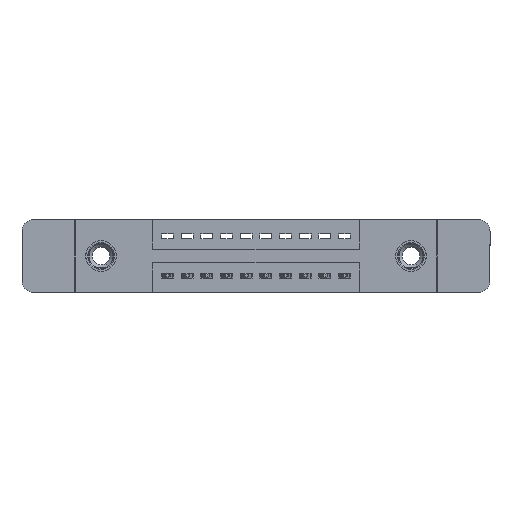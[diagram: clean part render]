
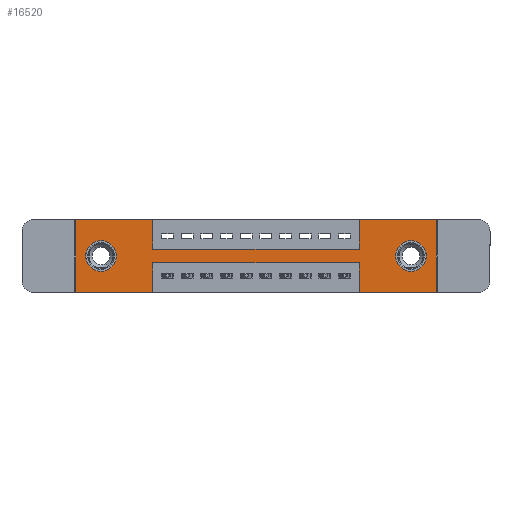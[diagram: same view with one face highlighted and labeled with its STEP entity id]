
A CAD part, front view. The second image highlights one B-rep face of the part: STEP entity #16520.
In plain terms, the highlighted planar face has unit normal (0, -1, 0).
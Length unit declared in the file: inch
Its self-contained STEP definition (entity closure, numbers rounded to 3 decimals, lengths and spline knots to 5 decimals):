
#127 = CARTESIAN_POINT ( 'NONE',  ( 0.3925, 0., 0. ) ) ;
#152 = ORIENTED_EDGE ( 'NONE', *, *, #13595, .F. ) ;
#207 = LINE ( 'NONE', #127, #14600 ) ;
#641 = EDGE_CURVE ( 'NONE', #5445, #3147, #5574, .T. ) ;
#910 = VECTOR ( 'NONE', #4102, 39.37008 ) ;
#1420 = CARTESIAN_POINT ( 'NONE',  ( 0.13, 0., -0.107 ) ) ;
#1727 = ORIENTED_EDGE ( 'NONE', *, *, #8128, .F. ) ;
#1842 = ORIENTED_EDGE ( 'NONE', *, *, #15267, .F. ) ;
#2027 = FACE_BOUND ( 'NONE', #13769, .T. ) ;
#2167 = CARTESIAN_POINT ( 'NONE',  ( 1.4425, 0., -0.37 ) ) ;
#2197 = ORIENTED_EDGE ( 'NONE', *, *, #5052, .F. ) ;
#2280 = VECTOR ( 'NONE', #5036, 39.37008 ) ;
#2352 = CARTESIAN_POINT ( 'NONE',  ( 0., 0., 0. ) ) ;
#2382 = EDGE_CURVE ( 'NONE', #8239, #11735, #10687, .T. ) ;
#2415 = CARTESIAN_POINT ( 'NONE',  ( 0.3925, 0., -0.22 ) ) ;
#2597 = DIRECTION ( 'NONE',  ( -1., 0., 0. ) ) ;
#2602 = VECTOR ( 'NONE', #4194, 39.37008 ) ;
#2706 = EDGE_CURVE ( 'NONE', #8130, #14684, #16845, .T. ) ;
#2824 = CARTESIAN_POINT ( 'NONE',  ( 0., 0., 0. ) ) ;
#2878 = CARTESIAN_POINT ( 'NONE',  ( 1.4425, 0., 0. ) ) ;
#2883 = CARTESIAN_POINT ( 'NONE',  ( 0.3925, 0., -0.37 ) ) ;
#3040 = CARTESIAN_POINT ( 'NONE',  ( 0.3925, 0., 0. ) ) ;
#3147 = VERTEX_POINT ( 'NONE', #8772 ) ;
#3227 = CARTESIAN_POINT ( 'NONE',  ( 1.4425, 0., 0. ) ) ;
#3385 = EDGE_CURVE ( 'NONE', #3861, #8239, #7311, .T. ) ;
#3504 = DIRECTION ( 'NONE',  ( 0., 1., 0. ) ) ;
#3509 = EDGE_CURVE ( 'NONE', #13160, #3861, #6315, .T. ) ;
#3531 = CIRCLE ( 'NONE', #13431, 0.078 ) ;
#3548 = LINE ( 'NONE', #14357, #6642 ) ;
#3686 = VECTOR ( 'NONE', #14288, 39.37008 ) ;
#3698 = ORIENTED_EDGE ( 'NONE', *, *, #14165, .F. ) ;
#3845 = DIRECTION ( 'NONE',  ( 0., 1., 0. ) ) ;
#3861 = VERTEX_POINT ( 'NONE', #3227 ) ;
#3905 = CARTESIAN_POINT ( 'NONE',  ( 1.705, 0., -0.107 ) ) ;
#4102 = DIRECTION ( 'NONE',  ( 1., 0., 0. ) ) ;
#4194 = DIRECTION ( 'NONE',  ( 0., 0., 1. ) ) ;
#4401 = AXIS2_PLACEMENT_3D ( 'NONE', #11737, #3845, #6508 ) ;
#4901 = DIRECTION ( 'NONE',  ( 0., 0., 1. ) ) ;
#4958 = VECTOR ( 'NONE', #14741, 39.37008 ) ;
#5036 = DIRECTION ( 'NONE',  ( 0., 0., 1. ) ) ;
#5052 = EDGE_CURVE ( 'NONE', #11735, #5445, #8006, .T. ) ;
#5140 = CARTESIAN_POINT ( 'NONE',  ( 0.3925, 0., -0.37 ) ) ;
#5337 = CARTESIAN_POINT ( 'NONE',  ( 1.705, 0., -0.263 ) ) ;
#5445 = VERTEX_POINT ( 'NONE', #9207 ) ;
#5574 = LINE ( 'NONE', #2167, #11156 ) ;
#5982 = AXIS2_PLACEMENT_3D ( 'NONE', #14582, #16015, #15901 ) ;
#6210 = CIRCLE ( 'NONE', #4401, 0.078 ) ;
#6250 = VERTEX_POINT ( 'NONE', #3040 ) ;
#6315 = LINE ( 'NONE', #2878, #2602 ) ;
#6354 = ORIENTED_EDGE ( 'NONE', *, *, #2382, .F. ) ;
#6387 = CARTESIAN_POINT ( 'NONE',  ( 0., 0., 0. ) ) ;
#6447 = ORIENTED_EDGE ( 'NONE', *, *, #2706, .F. ) ;
#6468 = DIRECTION ( 'NONE',  ( 0., 1., 0. ) ) ;
#6508 = DIRECTION ( 'NONE',  ( 0., 0., -1. ) ) ;
#6642 = VECTOR ( 'NONE', #2597, 39.37008 ) ;
#7075 = CARTESIAN_POINT ( 'NONE',  ( 0.13, 0., -0.185 ) ) ;
#7215 = LINE ( 'NONE', #2824, #4958 ) ;
#7311 = LINE ( 'NONE', #6387, #10655 ) ;
#7471 = ORIENTED_EDGE ( 'NONE', *, *, #9266, .F. ) ;
#7651 = ORIENTED_EDGE ( 'NONE', *, *, #9530, .T. ) ;
#7866 = EDGE_CURVE ( 'NONE', #9955, #15402, #9528, .T. ) ;
#7925 = DIRECTION ( 'NONE',  ( 0., 0., -1. ) ) ;
#8006 = LINE ( 'NONE', #9879, #11098 ) ;
#8054 = DIRECTION ( 'NONE',  ( 0., 0., -1. ) ) ;
#8111 = AXIS2_PLACEMENT_3D ( 'NONE', #14363, #6468, #9265 ) ;
#8128 = EDGE_CURVE ( 'NONE', #11475, #13160, #12873, .T. ) ;
#8130 = VERTEX_POINT ( 'NONE', #14544 ) ;
#8239 = VERTEX_POINT ( 'NONE', #14656 ) ;
#8362 = EDGE_LOOP ( 'NONE', ( #13503, #11349 ) ) ;
#8706 = VERTEX_POINT ( 'NONE', #12957 ) ;
#8772 = CARTESIAN_POINT ( 'NONE',  ( 1.4425, 0., -0.22 ) ) ;
#9207 = CARTESIAN_POINT ( 'NONE',  ( 1.4425, 0., -0.37 ) ) ;
#9265 = DIRECTION ( 'NONE',  ( 0., 0., 1. ) ) ;
#9266 = EDGE_CURVE ( 'NONE', #14684, #8706, #3548, .T. ) ;
#9275 = VERTEX_POINT ( 'NONE', #5337 ) ;
#9420 = LINE ( 'NONE', #2415, #3686 ) ;
#9528 = CIRCLE ( 'NONE', #8111, 0.078 ) ;
#9530 = EDGE_CURVE ( 'NONE', #12639, #9275, #3531, .T. ) ;
#9879 = CARTESIAN_POINT ( 'NONE',  ( 0., 0., -0.37 ) ) ;
#9925 = VERTEX_POINT ( 'NONE', #14565 ) ;
#9955 = VERTEX_POINT ( 'NONE', #1420 ) ;
#10281 = CARTESIAN_POINT ( 'NONE',  ( 1.4425, 0., -0.15 ) ) ;
#10358 = DIRECTION ( 'NONE',  ( 1., 0., 0. ) ) ;
#10365 = CARTESIAN_POINT ( 'NONE',  ( 1.835, 0., 0. ) ) ;
#10467 = VECTOR ( 'NONE', #8054, 39.37008 ) ;
#10655 = VECTOR ( 'NONE', #10358, 39.37008 ) ;
#10687 = LINE ( 'NONE', #10365, #11513 ) ;
#10866 = CARTESIAN_POINT ( 'NONE',  ( 0.13, 0., -0.263 ) ) ;
#10874 = FACE_OUTER_BOUND ( 'NONE', #14163, .T. ) ;
#11098 = VECTOR ( 'NONE', #16309, 39.37008 ) ;
#11156 = VECTOR ( 'NONE', #15187, 39.37008 ) ;
#11282 = CARTESIAN_POINT ( 'NONE',  ( 1.705, 0., -0.185 ) ) ;
#11349 = ORIENTED_EDGE ( 'NONE', *, *, #14623, .T. ) ;
#11475 = VERTEX_POINT ( 'NONE', #14987 ) ;
#11513 = VECTOR ( 'NONE', #15964, 39.37008 ) ;
#11735 = VERTEX_POINT ( 'NONE', #13826 ) ;
#11737 = CARTESIAN_POINT ( 'NONE',  ( 1.705, 0., -0.185 ) ) ;
#11881 = CARTESIAN_POINT ( 'NONE',  ( 0.3925, 0., -0.15 ) ) ;
#11967 = ORIENTED_EDGE ( 'NONE', *, *, #13572, .T. ) ;
#12164 = AXIS2_PLACEMENT_3D ( 'NONE', #7075, #12769, #4901 ) ;
#12527 = ORIENTED_EDGE ( 'NONE', *, *, #641, .F. ) ;
#12639 = VERTEX_POINT ( 'NONE', #3905 ) ;
#12769 = DIRECTION ( 'NONE',  ( 0., 1., 0. ) ) ;
#12873 = LINE ( 'NONE', #11881, #910 ) ;
#12957 = CARTESIAN_POINT ( 'NONE',  ( 0., 0., -0.37 ) ) ;
#13128 = ORIENTED_EDGE ( 'NONE', *, *, #3509, .F. ) ;
#13160 = VERTEX_POINT ( 'NONE', #10281 ) ;
#13382 = ORIENTED_EDGE ( 'NONE', *, *, #15000, .F. ) ;
#13431 = AXIS2_PLACEMENT_3D ( 'NONE', #11282, #3504, #16512 ) ;
#13503 = ORIENTED_EDGE ( 'NONE', *, *, #7866, .T. ) ;
#13572 = EDGE_CURVE ( 'NONE', #9275, #12639, #6210, .T. ) ;
#13595 = EDGE_CURVE ( 'NONE', #9925, #6250, #7215, .T. ) ;
#13769 = EDGE_LOOP ( 'NONE', ( #7651, #11967 ) ) ;
#13826 = CARTESIAN_POINT ( 'NONE',  ( 1.835, 0., -0.37 ) ) ;
#14163 = EDGE_LOOP ( 'NONE', ( #6447, #13382, #12527, #2197, #6354, #16338, #13128, #1727, #1842, #152, #3698, #7471 ) ) ;
#14165 = EDGE_CURVE ( 'NONE', #8706, #9925, #15061, .T. ) ;
#14288 = DIRECTION ( 'NONE',  ( -1., 0., 0. ) ) ;
#14357 = CARTESIAN_POINT ( 'NONE',  ( 0., 0., -0.37 ) ) ;
#14363 = CARTESIAN_POINT ( 'NONE',  ( 0.13, 0., -0.185 ) ) ;
#14544 = CARTESIAN_POINT ( 'NONE',  ( 0.3925, 0., -0.22 ) ) ;
#14565 = CARTESIAN_POINT ( 'NONE',  ( 0., 0., 0. ) ) ;
#14582 = CARTESIAN_POINT ( 'NONE',  ( 0., 0., -0.37 ) ) ;
#14600 = VECTOR ( 'NONE', #7925, 39.37008 ) ;
#14623 = EDGE_CURVE ( 'NONE', #15402, #9955, #15460, .T. ) ;
#14656 = CARTESIAN_POINT ( 'NONE',  ( 1.835, 0., 0. ) ) ;
#14684 = VERTEX_POINT ( 'NONE', #5140 ) ;
#14698 = PLANE ( 'NONE',  #5982 ) ;
#14741 = DIRECTION ( 'NONE',  ( 1., 0., 0. ) ) ;
#14987 = CARTESIAN_POINT ( 'NONE',  ( 0.3925, 0., -0.15 ) ) ;
#15000 = EDGE_CURVE ( 'NONE', #3147, #8130, #9420, .T. ) ;
#15061 = LINE ( 'NONE', #2352, #2280 ) ;
#15187 = DIRECTION ( 'NONE',  ( 0., 0., 1. ) ) ;
#15267 = EDGE_CURVE ( 'NONE', #6250, #11475, #207, .T. ) ;
#15402 = VERTEX_POINT ( 'NONE', #10866 ) ;
#15460 = CIRCLE ( 'NONE', #12164, 0.078 ) ;
#15901 = DIRECTION ( 'NONE',  ( 0., 0., -1. ) ) ;
#15964 = DIRECTION ( 'NONE',  ( 0., 0., -1. ) ) ;
#16015 = DIRECTION ( 'NONE',  ( 0., -1., 0. ) ) ;
#16233 = FACE_BOUND ( 'NONE', #8362, .T. ) ;
#16309 = DIRECTION ( 'NONE',  ( -1., 0., 0. ) ) ;
#16338 = ORIENTED_EDGE ( 'NONE', *, *, #3385, .F. ) ;
#16512 = DIRECTION ( 'NONE',  ( 0., 0., -1. ) ) ;
#16520 = ADVANCED_FACE ( 'NONE', ( #2027, #16233, #10874 ), #14698, .T. ) ;
#16845 = LINE ( 'NONE', #2883, #10467 ) ;
